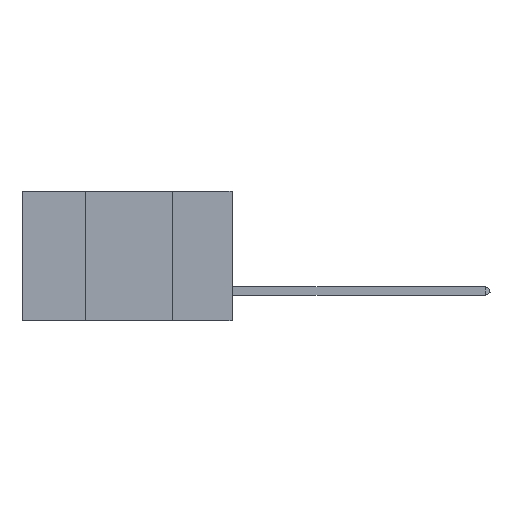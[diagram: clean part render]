
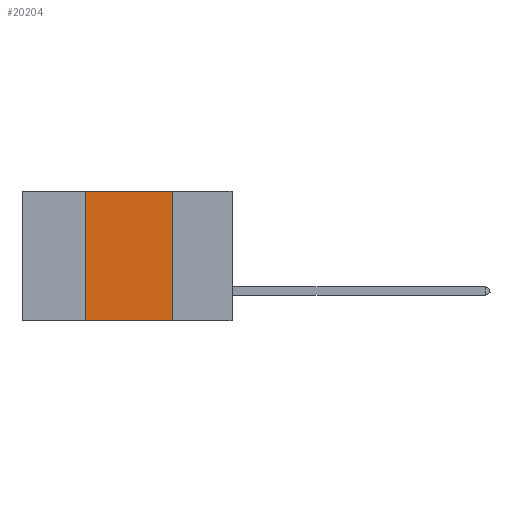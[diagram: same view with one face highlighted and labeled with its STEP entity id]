
A CAD part, left-side view. The second image highlights one B-rep face of the part: STEP entity #20204.
In plain terms, the highlighted planar face has unit normal (-1, 0, 0).
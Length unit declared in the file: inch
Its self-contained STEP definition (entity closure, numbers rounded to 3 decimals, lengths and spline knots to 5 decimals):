
#1311 = DIRECTION ( 'NONE',  ( 0., 0., -1. ) ) ;
#1376 = CARTESIAN_POINT ( 'NONE',  ( 0., 0.42, 0. ) ) ;
#2833 = VERTEX_POINT ( 'NONE', #1376 ) ;
#4312 = CARTESIAN_POINT ( 'NONE',  ( 0., 0.42, -0.37 ) ) ;
#5789 = CARTESIAN_POINT ( 'NONE',  ( 0., 0.17, -0.37 ) ) ;
#5990 = EDGE_CURVE ( 'NONE', #2833, #12261, #22335, .T. ) ;
#8568 = ORIENTED_EDGE ( 'NONE', *, *, #5990, .F. ) ;
#8589 = DIRECTION ( 'NONE',  ( 0., 0., -1. ) ) ;
#8723 = DIRECTION ( 'NONE',  ( 0., -1., 0. ) ) ;
#9089 = DIRECTION ( 'NONE',  ( 0., 0., 1. ) ) ;
#11688 = VECTOR ( 'NONE', #9089, 39.37008 ) ;
#12261 = VERTEX_POINT ( 'NONE', #23133 ) ;
#12302 = ORIENTED_EDGE ( 'NONE', *, *, #20926, .T. ) ;
#13398 = EDGE_LOOP ( 'NONE', ( #25780, #8568, #21903, #12302 ) ) ;
#14394 = LINE ( 'NONE', #24897, #22000 ) ;
#14719 = PLANE ( 'NONE',  #27292 ) ;
#16058 = CARTESIAN_POINT ( 'NONE',  ( 0., 0.17, 0. ) ) ;
#16844 = CARTESIAN_POINT ( 'NONE',  ( 0., 0.6, 0. ) ) ;
#17669 = LINE ( 'NONE', #22143, #11688 ) ;
#18746 = FACE_OUTER_BOUND ( 'NONE', #13398, .T. ) ;
#19413 = EDGE_CURVE ( 'NONE', #12261, #27376, #21883, .T. ) ;
#20204 = ADVANCED_FACE ( 'NONE', ( #18746 ), #14719, .F. ) ;
#20463 = DIRECTION ( 'NONE',  ( 0., -1., 0. ) ) ;
#20926 = EDGE_CURVE ( 'NONE', #21225, #27376, #14394, .T. ) ;
#21107 = DIRECTION ( 'NONE',  ( 1., 0., 0. ) ) ;
#21225 = VERTEX_POINT ( 'NONE', #4312 ) ;
#21883 = LINE ( 'NONE', #16058, #26854 ) ;
#21903 = ORIENTED_EDGE ( 'NONE', *, *, #21973, .F. ) ;
#21973 = EDGE_CURVE ( 'NONE', #21225, #2833, #17669, .T. ) ;
#22000 = VECTOR ( 'NONE', #20463, 39.37008 ) ;
#22143 = CARTESIAN_POINT ( 'NONE',  ( 0., 0.42, 0. ) ) ;
#22335 = LINE ( 'NONE', #25839, #25683 ) ;
#23133 = CARTESIAN_POINT ( 'NONE',  ( 0., 0.17, 0. ) ) ;
#24897 = CARTESIAN_POINT ( 'NONE',  ( 0., 0.6, -0.37 ) ) ;
#25683 = VECTOR ( 'NONE', #8723, 39.37008 ) ;
#25780 = ORIENTED_EDGE ( 'NONE', *, *, #19413, .F. ) ;
#25839 = CARTESIAN_POINT ( 'NONE',  ( 0., 0.6, 0. ) ) ;
#26854 = VECTOR ( 'NONE', #1311, 39.37008 ) ;
#27292 = AXIS2_PLACEMENT_3D ( 'NONE', #16844, #21107, #8589 ) ;
#27376 = VERTEX_POINT ( 'NONE', #5789 ) ;
